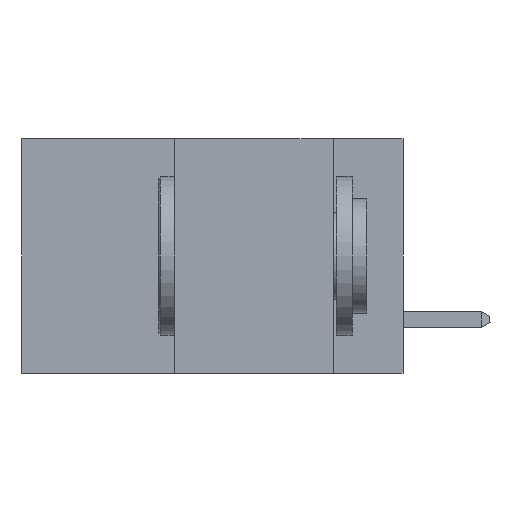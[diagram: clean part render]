
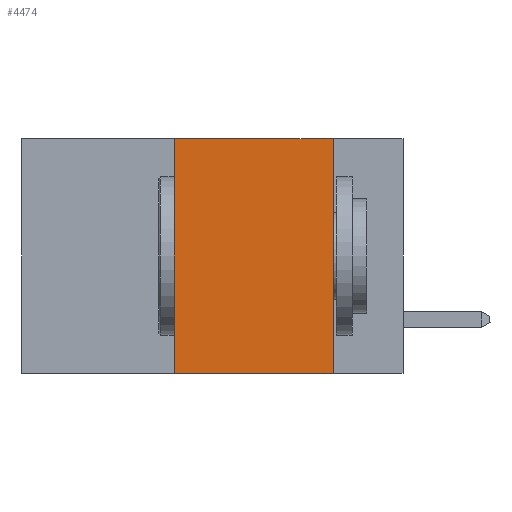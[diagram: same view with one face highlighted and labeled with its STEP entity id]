
A CAD part, left-side view. The second image highlights one B-rep face of the part: STEP entity #4474.
In plain terms, the highlighted planar face has unit normal (-1, 0, 0).
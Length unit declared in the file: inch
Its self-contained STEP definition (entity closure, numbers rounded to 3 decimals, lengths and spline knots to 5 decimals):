
#735 = LINE ( 'NONE', #4485, #12824 ) ;
#1982 = ORIENTED_EDGE ( 'NONE', *, *, #11077, .F. ) ;
#2526 = VERTEX_POINT ( 'NONE', #10087 ) ;
#2876 = EDGE_CURVE ( 'NONE', #6173, #2526, #735, .T. ) ;
#2938 = EDGE_CURVE ( 'NONE', #12857, #6173, #3203, .T. ) ;
#3044 = CARTESIAN_POINT ( 'NONE',  ( 0., 0.36, -0.37 ) ) ;
#3083 = EDGE_CURVE ( 'NONE', #7888, #2526, #8825, .T. ) ;
#3203 = LINE ( 'NONE', #5852, #5084 ) ;
#4140 = CARTESIAN_POINT ( 'NONE',  ( 0., 0.11, 0. ) ) ;
#4474 = ADVANCED_FACE ( 'NONE', ( #6076 ), #9867, .F. ) ;
#4485 = CARTESIAN_POINT ( 'NONE',  ( 0., 0.11, 0. ) ) ;
#5084 = VECTOR ( 'NONE', #8068, 39.37008 ) ;
#5093 = CARTESIAN_POINT ( 'NONE',  ( 0., 0.36, 0. ) ) ;
#5182 = CARTESIAN_POINT ( 'NONE',  ( 0., 0.6, -0.37 ) ) ;
#5685 = CARTESIAN_POINT ( 'NONE',  ( 0., 0.6, 0. ) ) ;
#5852 = CARTESIAN_POINT ( 'NONE',  ( 0., 0.6, 0. ) ) ;
#6076 = FACE_OUTER_BOUND ( 'NONE', #10659, .T. ) ;
#6173 = VERTEX_POINT ( 'NONE', #4140 ) ;
#6188 = DIRECTION ( 'NONE',  ( 0., 0., 1. ) ) ;
#7067 = DIRECTION ( 'NONE',  ( 0., 0., -1. ) ) ;
#7369 = DIRECTION ( 'NONE',  ( 0., -1., 0. ) ) ;
#7832 = LINE ( 'NONE', #12579, #10023 ) ;
#7888 = VERTEX_POINT ( 'NONE', #3044 ) ;
#8068 = DIRECTION ( 'NONE',  ( 0., -1., 0. ) ) ;
#8773 = ORIENTED_EDGE ( 'NONE', *, *, #2876, .F. ) ;
#8825 = LINE ( 'NONE', #5182, #12493 ) ;
#9383 = AXIS2_PLACEMENT_3D ( 'NONE', #5685, #11945, #11199 ) ;
#9867 = PLANE ( 'NONE',  #9383 ) ;
#10023 = VECTOR ( 'NONE', #6188, 39.37008 ) ;
#10087 = CARTESIAN_POINT ( 'NONE',  ( 0., 0.11, -0.37 ) ) ;
#10659 = EDGE_LOOP ( 'NONE', ( #8773, #12159, #1982, #13544 ) ) ;
#11077 = EDGE_CURVE ( 'NONE', #7888, #12857, #7832, .T. ) ;
#11199 = DIRECTION ( 'NONE',  ( 0., 0., -1. ) ) ;
#11945 = DIRECTION ( 'NONE',  ( 1., 0., 0. ) ) ;
#12159 = ORIENTED_EDGE ( 'NONE', *, *, #2938, .F. ) ;
#12493 = VECTOR ( 'NONE', #7369, 39.37008 ) ;
#12579 = CARTESIAN_POINT ( 'NONE',  ( 0., 0.36, 0. ) ) ;
#12824 = VECTOR ( 'NONE', #7067, 39.37008 ) ;
#12857 = VERTEX_POINT ( 'NONE', #5093 ) ;
#13544 = ORIENTED_EDGE ( 'NONE', *, *, #3083, .T. ) ;
